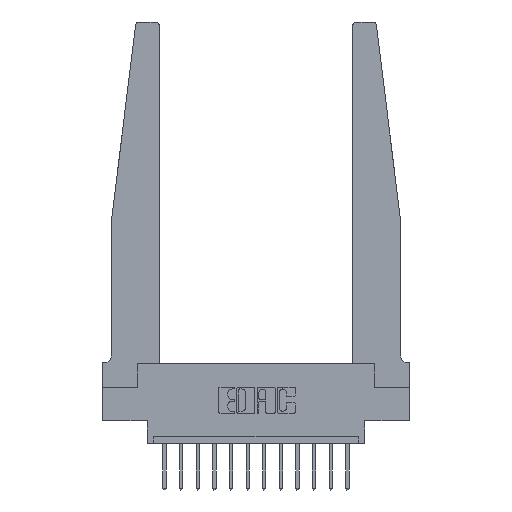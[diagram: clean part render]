
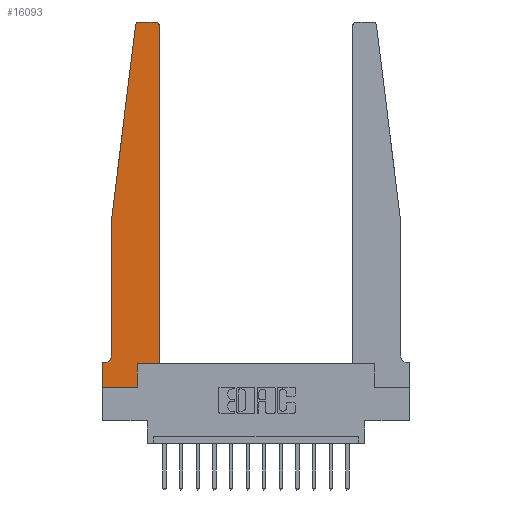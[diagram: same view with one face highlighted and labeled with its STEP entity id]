
A CAD part, top view. The second image highlights one B-rep face of the part: STEP entity #16093.
In plain terms, the highlighted planar face has unit normal (0, 0, 1).
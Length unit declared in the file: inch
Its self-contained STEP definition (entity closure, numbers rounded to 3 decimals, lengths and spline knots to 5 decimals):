
#230 = AXIS2_PLACEMENT_3D ( 'NONE', #2150, #4773, #11075 ) ;
#527 = LINE ( 'NONE', #13524, #12050 ) ;
#543 = CARTESIAN_POINT ( 'NONE',  ( 0.395, 2.75, 0.37 ) ) ;
#554 = ORIENTED_EDGE ( 'NONE', *, *, #6742, .T. ) ;
#605 = LINE ( 'NONE', #849, #14348 ) ;
#849 = CARTESIAN_POINT ( 'NONE',  ( 0.2605, 0.18, 0.37 ) ) ;
#1209 = ORIENTED_EDGE ( 'NONE', *, *, #7387, .T. ) ;
#1212 = CARTESIAN_POINT ( 'NONE',  ( 0., 0., 0.37 ) ) ;
#1286 = CIRCLE ( 'NONE', #2929, 0.03 ) ;
#1529 = VECTOR ( 'NONE', #6948, 39.37008 ) ;
#1650 = DIRECTION ( 'NONE',  ( 1., 0., 0. ) ) ;
#1738 = VERTEX_POINT ( 'NONE', #10224 ) ;
#1752 = EDGE_CURVE ( 'NONE', #14907, #1738, #4035, .T. ) ;
#1755 = EDGE_CURVE ( 'NONE', #3651, #2182, #9286, .T. ) ;
#1791 = VERTEX_POINT ( 'NONE', #9208 ) ;
#2044 = CARTESIAN_POINT ( 'NONE',  ( 0.25, 2.75, 0.37 ) ) ;
#2150 = CARTESIAN_POINT ( 'NONE',  ( 0., 0.1875, 0.37 ) ) ;
#2182 = VERTEX_POINT ( 'NONE', #2313 ) ;
#2313 = CARTESIAN_POINT ( 'NONE',  ( 0.2605, 0., 0.37 ) ) ;
#2515 = VERTEX_POINT ( 'NONE', #3206 ) ;
#2611 = DIRECTION ( 'NONE',  ( -1., 0., 0. ) ) ;
#2929 = AXIS2_PLACEMENT_3D ( 'NONE', #7535, #16237, #5931 ) ;
#2978 = LINE ( 'NONE', #1212, #11343 ) ;
#3206 = CARTESIAN_POINT ( 'NONE',  ( 0.425, 0.18, 0.37 ) ) ;
#3443 = ORIENTED_EDGE ( 'NONE', *, *, #9017, .T. ) ;
#3651 = VERTEX_POINT ( 'NONE', #9010 ) ;
#4035 = LINE ( 'NONE', #7838, #16075 ) ;
#4133 = CARTESIAN_POINT ( 'NONE',  ( 0.065, 0.1875, 0.37 ) ) ;
#4773 = DIRECTION ( 'NONE',  ( 0., 0., 1. ) ) ;
#4834 = DIRECTION ( 'NONE',  ( 0., 0., 1. ) ) ;
#4961 = ORIENTED_EDGE ( 'NONE', *, *, #13065, .T. ) ;
#5296 = DIRECTION ( 'NONE',  ( 0., -1., 0. ) ) ;
#5322 = VECTOR ( 'NONE', #7320, 39.37008 ) ;
#5422 = ORIENTED_EDGE ( 'NONE', *, *, #1752, .T. ) ;
#5483 = EDGE_CURVE ( 'NONE', #1791, #5812, #1286, .T. ) ;
#5683 = EDGE_CURVE ( 'NONE', #1738, #6982, #14050, .T. ) ;
#5789 = DIRECTION ( 'NONE',  ( 0., 1., 0. ) ) ;
#5809 = LINE ( 'NONE', #16445, #10524 ) ;
#5812 = VERTEX_POINT ( 'NONE', #12036 ) ;
#5931 = DIRECTION ( 'NONE',  ( 1., 0., 0. ) ) ;
#6277 = CARTESIAN_POINT ( 'NONE',  ( 0.065, 1.25, 0.37 ) ) ;
#6339 = CARTESIAN_POINT ( 'NONE',  ( 0.015, 0.2375, 0.37 ) ) ;
#6355 = CARTESIAN_POINT ( 'NONE',  ( 0.015, 0.1875, 0.37 ) ) ;
#6395 = EDGE_CURVE ( 'NONE', #5812, #14907, #5809, .T. ) ;
#6402 = DIRECTION ( 'NONE',  ( 1., 0., 0. ) ) ;
#6471 = VERTEX_POINT ( 'NONE', #16532 ) ;
#6495 = CARTESIAN_POINT ( 'NONE',  ( 0.395, 2.72, 0.37 ) ) ;
#6638 = ORIENTED_EDGE ( 'NONE', *, *, #6395, .T. ) ;
#6742 = EDGE_CURVE ( 'NONE', #2182, #6471, #605, .T. ) ;
#6948 = DIRECTION ( 'NONE',  ( -1., 0., 0. ) ) ;
#6982 = VERTEX_POINT ( 'NONE', #6355 ) ;
#7320 = DIRECTION ( 'NONE',  ( 0., 1., 0. ) ) ;
#7387 = EDGE_CURVE ( 'NONE', #12538, #12677, #11230, .T. ) ;
#7535 = CARTESIAN_POINT ( 'NONE',  ( 0.27653, 2.72, 0.37 ) ) ;
#7639 = ORIENTED_EDGE ( 'NONE', *, *, #14203, .T. ) ;
#7688 = DIRECTION ( 'NONE',  ( -1., 0., 0. ) ) ;
#7838 = CARTESIAN_POINT ( 'NONE',  ( 0.065, 1.25, 0.37 ) ) ;
#7956 = ORIENTED_EDGE ( 'NONE', *, *, #5483, .T. ) ;
#7996 = CARTESIAN_POINT ( 'NONE',  ( 0., 0., 0.37 ) ) ;
#8480 = CARTESIAN_POINT ( 'NONE',  ( 0., 0.1875, 0.37 ) ) ;
#8652 = ORIENTED_EDGE ( 'NONE', *, *, #11903, .T. ) ;
#8704 = VERTEX_POINT ( 'NONE', #8480 ) ;
#9010 = CARTESIAN_POINT ( 'NONE',  ( 0., 0., 0.37 ) ) ;
#9017 = EDGE_CURVE ( 'NONE', #2515, #12538, #9798, .T. ) ;
#9208 = CARTESIAN_POINT ( 'NONE',  ( 0.27653, 2.75, 0.37 ) ) ;
#9270 = VECTOR ( 'NONE', #1650, 39.37008 ) ;
#9286 = LINE ( 'NONE', #7996, #9270 ) ;
#9798 = LINE ( 'NONE', #12428, #5322 ) ;
#10224 = CARTESIAN_POINT ( 'NONE',  ( 0.065, 0.2375, 0.37 ) ) ;
#10524 = VECTOR ( 'NONE', #11172, 39.37008 ) ;
#10680 = AXIS2_PLACEMENT_3D ( 'NONE', #6495, #4834, #6402 ) ;
#11075 = DIRECTION ( 'NONE',  ( 1., 0., 0. ) ) ;
#11172 = DIRECTION ( 'NONE',  ( -0.122, -0.992, 0. ) ) ;
#11230 = CIRCLE ( 'NONE', #10680, 0.03 ) ;
#11238 = PLANE ( 'NONE',  #230 ) ;
#11343 = VECTOR ( 'NONE', #16006, 39.37008 ) ;
#11543 = DIRECTION ( 'NONE',  ( 0., 0., -1. ) ) ;
#11606 = VECTOR ( 'NONE', #7688, 39.37008 ) ;
#11633 = ORIENTED_EDGE ( 'NONE', *, *, #1755, .T. ) ;
#11903 = EDGE_CURVE ( 'NONE', #6471, #2515, #527, .T. ) ;
#11928 = CARTESIAN_POINT ( 'NONE',  ( 0.425, 2.72, 0.37 ) ) ;
#12036 = CARTESIAN_POINT ( 'NONE',  ( 0.24675, 2.72367, 0.37 ) ) ;
#12050 = VECTOR ( 'NONE', #13434, 39.37008 ) ;
#12428 = CARTESIAN_POINT ( 'NONE',  ( 0.425, 0.18, 0.37 ) ) ;
#12538 = VERTEX_POINT ( 'NONE', #11928 ) ;
#12677 = VERTEX_POINT ( 'NONE', #543 ) ;
#12877 = LINE ( 'NONE', #4133, #11606 ) ;
#13065 = EDGE_CURVE ( 'NONE', #12677, #1791, #15054, .T. ) ;
#13434 = DIRECTION ( 'NONE',  ( 1., 0., 0. ) ) ;
#13524 = CARTESIAN_POINT ( 'NONE',  ( 0.425, 0.18, 0.37 ) ) ;
#13791 = FACE_OUTER_BOUND ( 'NONE', #15710, .T. ) ;
#13867 = ORIENTED_EDGE ( 'NONE', *, *, #5683, .T. ) ;
#14050 = CIRCLE ( 'NONE', #15965, 0.05 ) ;
#14203 = EDGE_CURVE ( 'NONE', #6982, #8704, #12877, .T. ) ;
#14348 = VECTOR ( 'NONE', #5789, 39.37008 ) ;
#14720 = EDGE_CURVE ( 'NONE', #8704, #3651, #2978, .T. ) ;
#14907 = VERTEX_POINT ( 'NONE', #6277 ) ;
#15054 = LINE ( 'NONE', #2044, #1529 ) ;
#15575 = ORIENTED_EDGE ( 'NONE', *, *, #14720, .T. ) ;
#15710 = EDGE_LOOP ( 'NONE', ( #4961, #7956, #6638, #5422, #13867, #7639, #15575, #11633, #554, #8652, #3443, #1209 ) ) ;
#15965 = AXIS2_PLACEMENT_3D ( 'NONE', #6339, #11543, #2611 ) ;
#16006 = DIRECTION ( 'NONE',  ( 0., -1., 0. ) ) ;
#16075 = VECTOR ( 'NONE', #5296, 39.37008 ) ;
#16093 = ADVANCED_FACE ( 'NONE', ( #13791 ), #11238, .T. ) ;
#16237 = DIRECTION ( 'NONE',  ( 0., 0., 1. ) ) ;
#16445 = CARTESIAN_POINT ( 'NONE',  ( 0.065, 1.25, 0.37 ) ) ;
#16532 = CARTESIAN_POINT ( 'NONE',  ( 0.2605, 0.18, 0.37 ) ) ;
